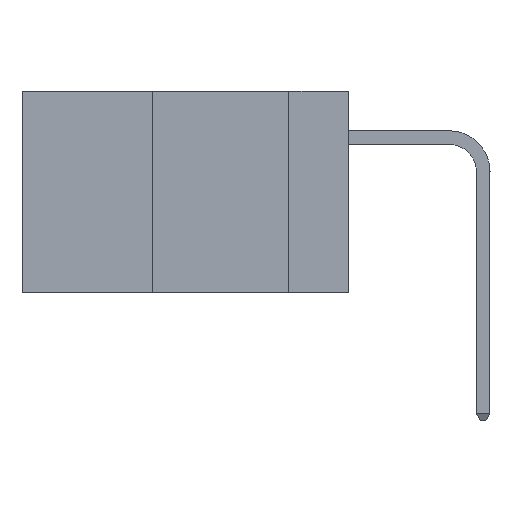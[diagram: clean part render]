
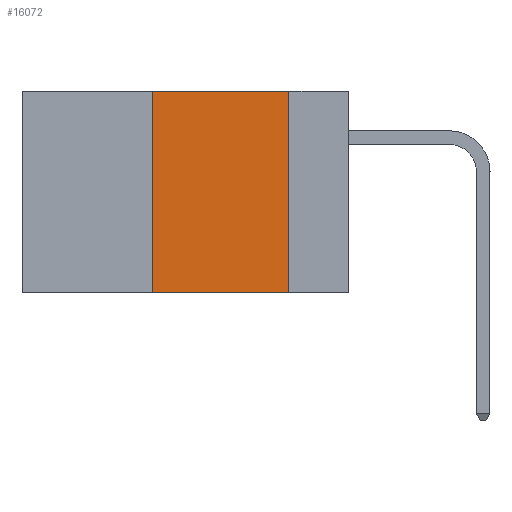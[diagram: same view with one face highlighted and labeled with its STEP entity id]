
A CAD part, left-side view. The second image highlights one B-rep face of the part: STEP entity #16072.
In plain terms, the highlighted planar face has unit normal (-1, 0, 0).
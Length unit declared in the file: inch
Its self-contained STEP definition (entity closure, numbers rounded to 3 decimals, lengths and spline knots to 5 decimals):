
#73 = AXIS2_PLACEMENT_3D ( 'NONE', #33931, #8091, #41647 ) ;
#257 = LINE ( 'NONE', #38425, #35315 ) ;
#2027 = ORIENTED_EDGE ( 'NONE', *, *, #36041, .T. ) ;
#2345 = FACE_OUTER_BOUND ( 'NONE', #6396, .T. ) ;
#3509 = CARTESIAN_POINT ( 'NONE',  ( 0., 0.11, 0. ) ) ;
#6396 = EDGE_LOOP ( 'NONE', ( #31641, #22709, #13009, #2027 ) ) ;
#6654 = DIRECTION ( 'NONE',  ( 0., -1., 0. ) ) ;
#6729 = VECTOR ( 'NONE', #29967, 39.37008 ) ;
#6959 = DIRECTION ( 'NONE',  ( 0., 0., 1. ) ) ;
#7266 = CARTESIAN_POINT ( 'NONE',  ( 0., 0.36, -0.37 ) ) ;
#7522 = EDGE_CURVE ( 'NONE', #25816, #27472, #16671, .T. ) ;
#8091 = DIRECTION ( 'NONE',  ( 1., 0., 0. ) ) ;
#8769 = EDGE_CURVE ( 'NONE', #48483, #16461, #21675, .T. ) ;
#10400 = CARTESIAN_POINT ( 'NONE',  ( 0., 0.6, 0. ) ) ;
#13009 = ORIENTED_EDGE ( 'NONE', *, *, #8769, .F. ) ;
#13941 = CARTESIAN_POINT ( 'NONE',  ( 0., 0.36, 0. ) ) ;
#15294 = PLANE ( 'NONE',  #73 ) ;
#15847 = EDGE_CURVE ( 'NONE', #16461, #25816, #39223, .T. ) ;
#16072 = ADVANCED_FACE ( 'NONE', ( #2345 ), #15294, .F. ) ;
#16461 = VERTEX_POINT ( 'NONE', #13941 ) ;
#16671 = LINE ( 'NONE', #3509, #6729 ) ;
#21675 = LINE ( 'NONE', #47903, #22848 ) ;
#22709 = ORIENTED_EDGE ( 'NONE', *, *, #15847, .F. ) ;
#22848 = VECTOR ( 'NONE', #6959, 39.37008 ) ;
#25816 = VERTEX_POINT ( 'NONE', #44841 ) ;
#27472 = VERTEX_POINT ( 'NONE', #40085 ) ;
#29272 = VECTOR ( 'NONE', #6654, 39.37008 ) ;
#29967 = DIRECTION ( 'NONE',  ( 0., 0., -1. ) ) ;
#31641 = ORIENTED_EDGE ( 'NONE', *, *, #7522, .F. ) ;
#33931 = CARTESIAN_POINT ( 'NONE',  ( 0., 0.6, 0. ) ) ;
#35315 = VECTOR ( 'NONE', #42515, 39.37008 ) ;
#36041 = EDGE_CURVE ( 'NONE', #48483, #27472, #257, .T. ) ;
#38425 = CARTESIAN_POINT ( 'NONE',  ( 0., 0.6, -0.37 ) ) ;
#39223 = LINE ( 'NONE', #10400, #29272 ) ;
#40085 = CARTESIAN_POINT ( 'NONE',  ( 0., 0.11, -0.37 ) ) ;
#41647 = DIRECTION ( 'NONE',  ( 0., 0., -1. ) ) ;
#42515 = DIRECTION ( 'NONE',  ( 0., -1., 0. ) ) ;
#44841 = CARTESIAN_POINT ( 'NONE',  ( 0., 0.11, 0. ) ) ;
#47903 = CARTESIAN_POINT ( 'NONE',  ( 0., 0.36, 0. ) ) ;
#48483 = VERTEX_POINT ( 'NONE', #7266 ) ;
